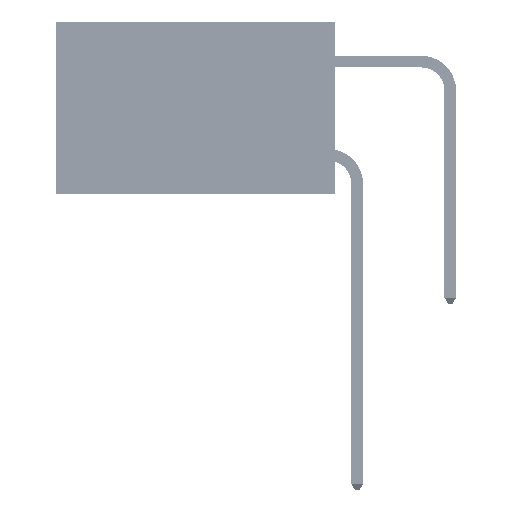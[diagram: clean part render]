
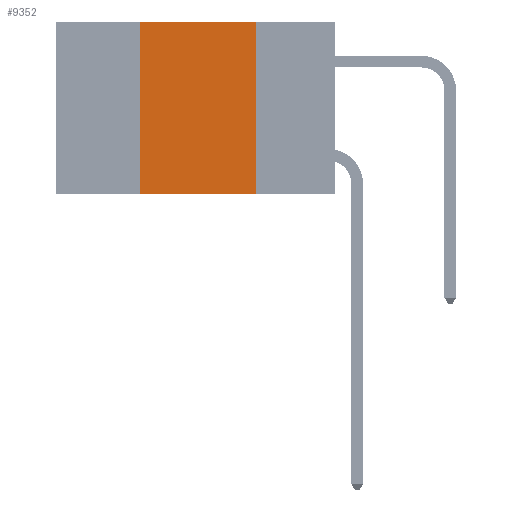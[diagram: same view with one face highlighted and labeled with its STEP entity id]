
A CAD part, left-side view. The second image highlights one B-rep face of the part: STEP entity #9352.
In plain terms, the highlighted planar face has unit normal (-1, 0, 0).
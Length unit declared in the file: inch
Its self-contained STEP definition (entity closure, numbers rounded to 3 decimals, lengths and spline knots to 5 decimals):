
#1528 = DIRECTION ( 'NONE',  ( 0., 0., 1. ) ) ;
#1796 = VECTOR ( 'NONE', #53721, 39.37008 ) ;
#4079 = EDGE_CURVE ( 'NONE', #24931, #31848, #40661, .T. ) ;
#4606 = LINE ( 'NONE', #9821, #52856 ) ;
#5397 = CARTESIAN_POINT ( 'NONE',  ( 0., 0.42, 0. ) ) ;
#5906 = ORIENTED_EDGE ( 'NONE', *, *, #29398, .T. ) ;
#5936 = CARTESIAN_POINT ( 'NONE',  ( 0., 0.17, 0. ) ) ;
#6914 = LINE ( 'NONE', #9577, #42686 ) ;
#9352 = ADVANCED_FACE ( 'NONE', ( #12489 ), #48696, .F. ) ;
#9577 = CARTESIAN_POINT ( 'NONE',  ( 0., 0.17, 0. ) ) ;
#9821 = CARTESIAN_POINT ( 'NONE',  ( 0., 0.6, -0.37 ) ) ;
#10038 = EDGE_LOOP ( 'NONE', ( #35685, #30446, #45048, #5906 ) ) ;
#10122 = DIRECTION ( 'NONE',  ( 0., 0., -1. ) ) ;
#12489 = FACE_OUTER_BOUND ( 'NONE', #10038, .T. ) ;
#15955 = CARTESIAN_POINT ( 'NONE',  ( 0., 0.6, 0. ) ) ;
#23008 = VERTEX_POINT ( 'NONE', #37512 ) ;
#24931 = VERTEX_POINT ( 'NONE', #52401 ) ;
#29398 = EDGE_CURVE ( 'NONE', #24931, #23008, #4606, .T. ) ;
#30446 = ORIENTED_EDGE ( 'NONE', *, *, #43819, .F. ) ;
#31839 = CARTESIAN_POINT ( 'NONE',  ( 0., 0.6, 0. ) ) ;
#31848 = VERTEX_POINT ( 'NONE', #5397 ) ;
#32212 = DIRECTION ( 'NONE',  ( 1., 0., 0. ) ) ;
#33407 = VECTOR ( 'NONE', #1528, 39.37008 ) ;
#35685 = ORIENTED_EDGE ( 'NONE', *, *, #50122, .F. ) ;
#37512 = CARTESIAN_POINT ( 'NONE',  ( 0., 0.17, -0.37 ) ) ;
#38230 = VERTEX_POINT ( 'NONE', #5936 ) ;
#40241 = LINE ( 'NONE', #15955, #1796 ) ;
#40661 = LINE ( 'NONE', #44125, #33407 ) ;
#42686 = VECTOR ( 'NONE', #10122, 39.37008 ) ;
#43364 = DIRECTION ( 'NONE',  ( 0., -1., 0. ) ) ;
#43819 = EDGE_CURVE ( 'NONE', #31848, #38230, #40241, .T. ) ;
#44125 = CARTESIAN_POINT ( 'NONE',  ( 0., 0.42, 0. ) ) ;
#45048 = ORIENTED_EDGE ( 'NONE', *, *, #4079, .F. ) ;
#48696 = PLANE ( 'NONE',  #48868 ) ;
#48868 = AXIS2_PLACEMENT_3D ( 'NONE', #31839, #32212, #53284 ) ;
#50122 = EDGE_CURVE ( 'NONE', #38230, #23008, #6914, .T. ) ;
#52401 = CARTESIAN_POINT ( 'NONE',  ( 0., 0.42, -0.37 ) ) ;
#52856 = VECTOR ( 'NONE', #43364, 39.37008 ) ;
#53284 = DIRECTION ( 'NONE',  ( 0., 0., -1. ) ) ;
#53721 = DIRECTION ( 'NONE',  ( 0., -1., 0. ) ) ;
